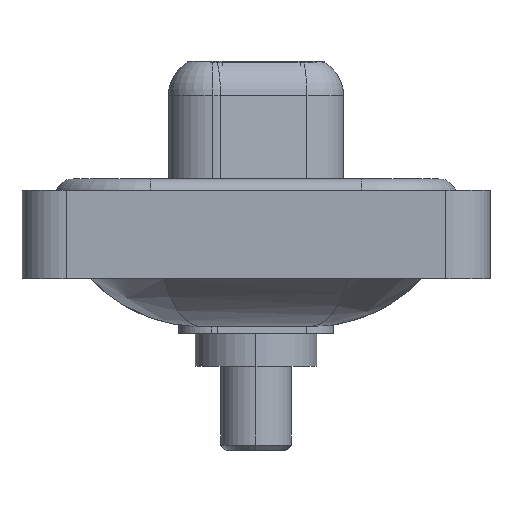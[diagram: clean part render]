
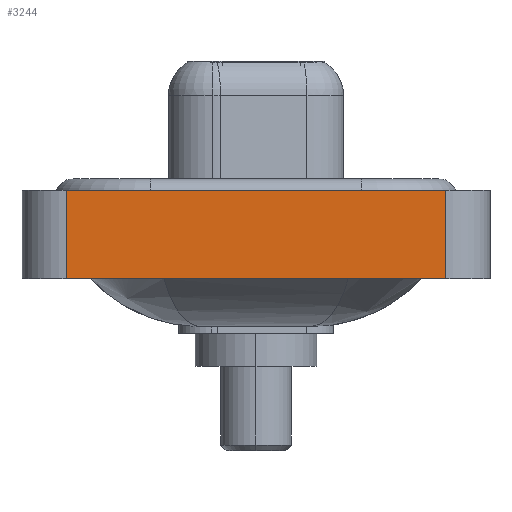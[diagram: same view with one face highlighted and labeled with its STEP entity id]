
A CAD part, left-side view. The second image highlights one B-rep face of the part: STEP entity #3244.
In plain terms, the highlighted planar face has unit normal (-1, 0, 0).
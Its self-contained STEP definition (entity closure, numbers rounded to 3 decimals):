
#949 = EDGE_CURVE ( 'NONE', #977, #15247, #8166, .T. ) ;
#977 = VERTEX_POINT ( 'NONE', #4385 ) ;
#1158 = ORIENTED_EDGE ( 'NONE', *, *, #3325, .F. ) ;
#1934 = EDGE_LOOP ( 'NONE', ( #7803, #1158, #4280, #2917 ) ) ;
#2917 = ORIENTED_EDGE ( 'NONE', *, *, #13287, .T. ) ;
#3244 = ADVANCED_FACE ( 'NONE', ( #14691 ), #11016, .T. ) ;
#3308 = DIRECTION ( 'NONE',  ( 0., 0., 1. ) ) ;
#3325 = EDGE_CURVE ( 'NONE', #11380, #15247, #8163, .T. ) ;
#3387 = LINE ( 'NONE', #15481, #6357 ) ;
#3538 = EDGE_CURVE ( 'NONE', #8170, #11380, #3387, .T. ) ;
#3663 = DIRECTION ( 'NONE',  ( 0., 0., 1. ) ) ;
#4280 = ORIENTED_EDGE ( 'NONE', *, *, #3538, .F. ) ;
#4385 = CARTESIAN_POINT ( 'NONE',  ( -7.3, -8.55, -3.6 ) ) ;
#4569 = CARTESIAN_POINT ( 'NONE',  ( -7.3, -8.55, -3.6 ) ) ;
#4700 = DIRECTION ( 'NONE',  ( 0., -1., 0. ) ) ;
#5209 = CARTESIAN_POINT ( 'NONE',  ( -7.3, 8.55, -3.6 ) ) ;
#5524 = CARTESIAN_POINT ( 'NONE',  ( -7.3, -8.55, -3.6 ) ) ;
#6077 = AXIS2_PLACEMENT_3D ( 'NONE', #4569, #11969, #3663 ) ;
#6357 = VECTOR ( 'NONE', #3308, 1000. ) ;
#6418 = LINE ( 'NONE', #15112, #8712 ) ;
#6890 = DIRECTION ( 'NONE',  ( 0., 0., 1. ) ) ;
#6996 = CARTESIAN_POINT ( 'NONE',  ( -7.3, 8.55, 0.4 ) ) ;
#7803 = ORIENTED_EDGE ( 'NONE', *, *, #949, .T. ) ;
#7861 = DIRECTION ( 'NONE',  ( 0., -1., 0. ) ) ;
#8163 = LINE ( 'NONE', #14500, #14539 ) ;
#8166 = LINE ( 'NONE', #5524, #10118 ) ;
#8170 = VERTEX_POINT ( 'NONE', #5209 ) ;
#8712 = VECTOR ( 'NONE', #7861, 1000. ) ;
#10118 = VECTOR ( 'NONE', #6890, 1000. ) ;
#11016 = PLANE ( 'NONE',  #6077 ) ;
#11380 = VERTEX_POINT ( 'NONE', #6996 ) ;
#11969 = DIRECTION ( 'NONE',  ( -1., 0., 0. ) ) ;
#12402 = CARTESIAN_POINT ( 'NONE',  ( -7.3, -8.55, 0.4 ) ) ;
#13287 = EDGE_CURVE ( 'NONE', #8170, #977, #6418, .T. ) ;
#14500 = CARTESIAN_POINT ( 'NONE',  ( -7.3, -8.55, 0.4 ) ) ;
#14539 = VECTOR ( 'NONE', #4700, 1000. ) ;
#14691 = FACE_OUTER_BOUND ( 'NONE', #1934, .T. ) ;
#15112 = CARTESIAN_POINT ( 'NONE',  ( -7.3, -8.55, -3.6 ) ) ;
#15247 = VERTEX_POINT ( 'NONE', #12402 ) ;
#15481 = CARTESIAN_POINT ( 'NONE',  ( -7.3, 8.55, -3.6 ) ) ;
